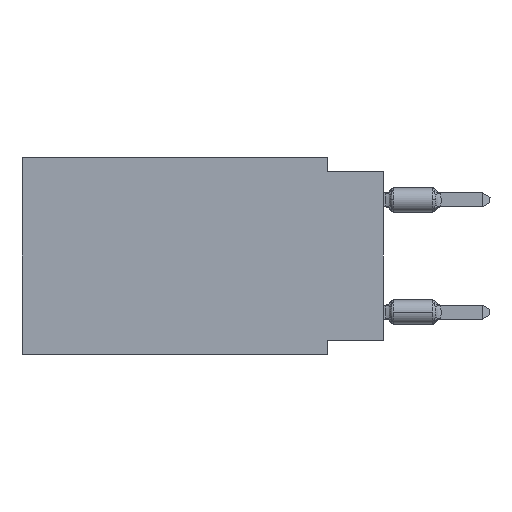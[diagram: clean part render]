
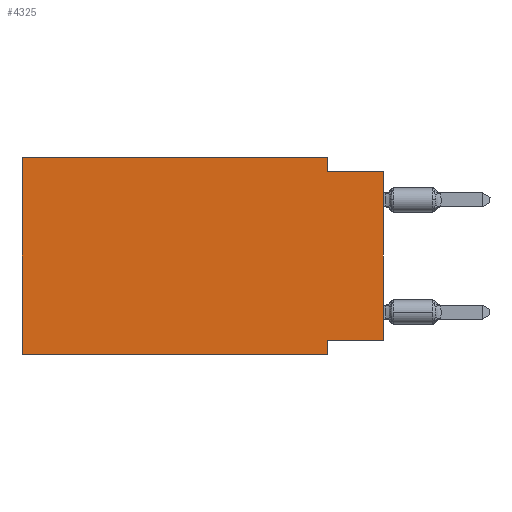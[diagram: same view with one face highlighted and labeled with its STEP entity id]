
A CAD part, left-side view. The second image highlights one B-rep face of the part: STEP entity #4325.
In plain terms, the highlighted planar face has unit normal (-1, 0, 0).
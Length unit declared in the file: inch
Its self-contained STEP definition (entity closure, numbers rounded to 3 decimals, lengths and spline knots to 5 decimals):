
#143 = ORIENTED_EDGE ( 'NONE', *, *, #9249, .T. ) ;
#514 = CARTESIAN_POINT ( 'NONE',  ( 0., 0.1, -0.35 ) ) ;
#879 = DIRECTION ( 'NONE',  ( 0., -1., 0. ) ) ;
#1026 = VERTEX_POINT ( 'NONE', #514 ) ;
#1549 = VERTEX_POINT ( 'NONE', #10879 ) ;
#1795 = FACE_OUTER_BOUND ( 'NONE', #6886, .T. ) ;
#2106 = CARTESIAN_POINT ( 'NONE',  ( 0., 0.645, 0. ) ) ;
#2145 = ORIENTED_EDGE ( 'NONE', *, *, #11441, .F. ) ;
#2358 = VECTOR ( 'NONE', #2594, 39.37008 ) ;
#2594 = DIRECTION ( 'NONE',  ( 0., 0., 1. ) ) ;
#2658 = DIRECTION ( 'NONE',  ( 0., 0., 1. ) ) ;
#2688 = EDGE_CURVE ( 'NONE', #11641, #1026, #6812, .T. ) ;
#2980 = CARTESIAN_POINT ( 'NONE',  ( 0., 0., -0.325 ) ) ;
#3133 = CARTESIAN_POINT ( 'NONE',  ( 0., 0.1, 0. ) ) ;
#3311 = DIRECTION ( 'NONE',  ( 1., 0., 0. ) ) ;
#3359 = DIRECTION ( 'NONE',  ( 0., -1., 0. ) ) ;
#4047 = CARTESIAN_POINT ( 'NONE',  ( 0., 0.1, -0.35 ) ) ;
#4060 = AXIS2_PLACEMENT_3D ( 'NONE', #16258, #3311, #9078 ) ;
#4325 = ADVANCED_FACE ( 'NONE', ( #1795 ), #17679, .F. ) ;
#4377 = DIRECTION ( 'NONE',  ( 0., 0., -1. ) ) ;
#4414 = CARTESIAN_POINT ( 'NONE',  ( 0., 0., -0.325 ) ) ;
#4568 = VERTEX_POINT ( 'NONE', #12707 ) ;
#4974 = CARTESIAN_POINT ( 'NONE',  ( 0., 0., -0.025 ) ) ;
#5455 = ORIENTED_EDGE ( 'NONE', *, *, #2688, .F. ) ;
#6118 = DIRECTION ( 'NONE',  ( 0., 1., 0. ) ) ;
#6174 = EDGE_CURVE ( 'NONE', #17197, #4568, #17122, .T. ) ;
#6784 = VERTEX_POINT ( 'NONE', #7706 ) ;
#6812 = LINE ( 'NONE', #4047, #10026 ) ;
#6844 = LINE ( 'NONE', #16938, #14266 ) ;
#6886 = EDGE_LOOP ( 'NONE', ( #143, #12385, #13486, #2145, #9268, #9515, #5455, #10834 ) ) ;
#7438 = LINE ( 'NONE', #4414, #7671 ) ;
#7671 = VECTOR ( 'NONE', #6118, 39.37008 ) ;
#7706 = CARTESIAN_POINT ( 'NONE',  ( 0., 0.645, -0.35 ) ) ;
#8315 = DIRECTION ( 'NONE',  ( 0., 0., -1. ) ) ;
#9078 = DIRECTION ( 'NONE',  ( 0., 0., -1. ) ) ;
#9249 = EDGE_CURVE ( 'NONE', #16367, #12616, #11019, .T. ) ;
#9268 = ORIENTED_EDGE ( 'NONE', *, *, #17023, .F. ) ;
#9515 = ORIENTED_EDGE ( 'NONE', *, *, #16312, .T. ) ;
#9985 = CARTESIAN_POINT ( 'NONE',  ( 0., 0.645, -0.35 ) ) ;
#10026 = VECTOR ( 'NONE', #8315, 39.37008 ) ;
#10834 = ORIENTED_EDGE ( 'NONE', *, *, #17695, .F. ) ;
#10879 = CARTESIAN_POINT ( 'NONE',  ( 0., 0.645, 0. ) ) ;
#11019 = LINE ( 'NONE', #13852, #2358 ) ;
#11430 = LINE ( 'NONE', #2106, #12761 ) ;
#11441 = EDGE_CURVE ( 'NONE', #1549, #17197, #11430, .T. ) ;
#11641 = VERTEX_POINT ( 'NONE', #13030 ) ;
#12385 = ORIENTED_EDGE ( 'NONE', *, *, #13064, .F. ) ;
#12616 = VERTEX_POINT ( 'NONE', #17844 ) ;
#12707 = CARTESIAN_POINT ( 'NONE',  ( 0., 0.1, -0.025 ) ) ;
#12761 = VECTOR ( 'NONE', #879, 39.37008 ) ;
#13030 = CARTESIAN_POINT ( 'NONE',  ( 0., 0.1, -0.325 ) ) ;
#13056 = VECTOR ( 'NONE', #15843, 39.37008 ) ;
#13064 = EDGE_CURVE ( 'NONE', #4568, #12616, #13653, .T. ) ;
#13486 = ORIENTED_EDGE ( 'NONE', *, *, #6174, .F. ) ;
#13653 = LINE ( 'NONE', #4974, #18243 ) ;
#13852 = CARTESIAN_POINT ( 'NONE',  ( 0., 0., 0. ) ) ;
#14266 = VECTOR ( 'NONE', #2658, 39.37008 ) ;
#14290 = CARTESIAN_POINT ( 'NONE',  ( 0., 0.1, 0. ) ) ;
#15843 = DIRECTION ( 'NONE',  ( 0., -1., 0. ) ) ;
#16258 = CARTESIAN_POINT ( 'NONE',  ( 0., 0.645, 0. ) ) ;
#16312 = EDGE_CURVE ( 'NONE', #6784, #1026, #18589, .T. ) ;
#16367 = VERTEX_POINT ( 'NONE', #2980 ) ;
#16938 = CARTESIAN_POINT ( 'NONE',  ( 0., 0.645, 0. ) ) ;
#17023 = EDGE_CURVE ( 'NONE', #6784, #1549, #6844, .T. ) ;
#17122 = LINE ( 'NONE', #14290, #18701 ) ;
#17197 = VERTEX_POINT ( 'NONE', #3133 ) ;
#17679 = PLANE ( 'NONE',  #4060 ) ;
#17695 = EDGE_CURVE ( 'NONE', #16367, #11641, #7438, .T. ) ;
#17844 = CARTESIAN_POINT ( 'NONE',  ( 0., 0., -0.025 ) ) ;
#18243 = VECTOR ( 'NONE', #3359, 39.37008 ) ;
#18589 = LINE ( 'NONE', #9985, #13056 ) ;
#18701 = VECTOR ( 'NONE', #4377, 39.37008 ) ;
